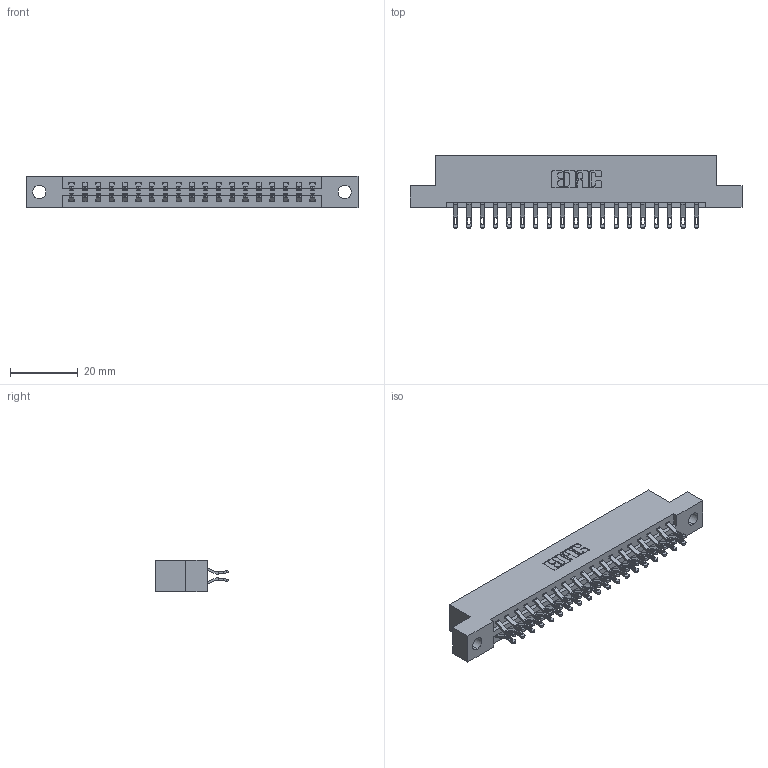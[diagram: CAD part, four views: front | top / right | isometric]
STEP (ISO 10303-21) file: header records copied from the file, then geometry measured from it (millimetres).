
FILE_DESCRIPTION (( 'STEP AP203' ), '1' );
FILE_NAME ('337-038-555-204.STEP', '2018-08-08T05:16:58', ( '' ), ( '' ), 'SwSTEP 2.0', 'SolidWorks 2016', '' );
FILE_SCHEMA (( 'CONFIG_CONTROL_DESIGN' ));
Length unit declared in the file: inch
Products named in the file (3): 337 Part_Flush Mounting Lugs - 0.156 Dia-TH; 345-292-001_555 Tail; 337-038-555-204
Assembly tree (39 placements, depth 2):
  337-038-555-204
    337 Part_Flush Mounting Lugs - 0.156 Dia-TH
    345-292-001_555 Tail  x38
Bounding box: 98.3 x 21.47 x 9.4 mm (x, y, z)
Volume: 10075.6 mm3; surface area: 11379.9 mm2
Topology: 39 solids, 39 shells, 2394 faces, 7493 edges, 4994 vertices
Faces by surface type: plane 1438, cylinder 956
Entity records: 18035 total; most frequent: CARTESIAN_POINT 3092, ORIENTED_EDGE 2998, DIRECTION 2643, EDGE_CURVE 1499, VECTOR 1351, LINE 1351, VERTEX_POINT 998, AXIS2_PLACEMENT_3D 646
